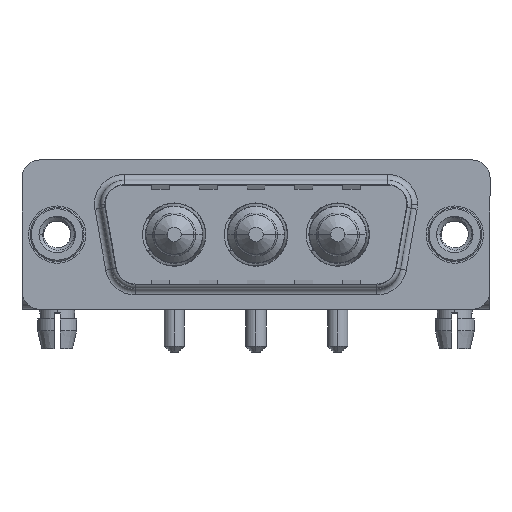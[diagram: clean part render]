
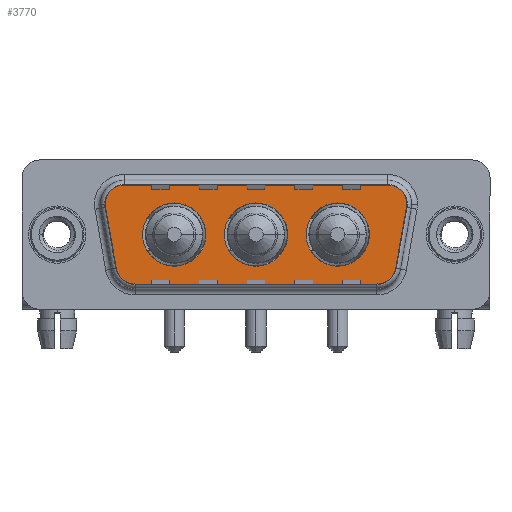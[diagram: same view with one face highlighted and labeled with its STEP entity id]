
A CAD part, top view. The second image highlights one B-rep face of the part: STEP entity #3770.
In plain terms, the highlighted planar face has unit normal (0, 0, 1).
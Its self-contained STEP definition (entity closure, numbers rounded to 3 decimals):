
#85 = ORIENTED_EDGE ( 'NONE', *, *, #2186, .F. ) ;
#625 = CARTESIAN_POINT ( 'NONE',  ( 9.8, 0., 0. ) ) ;
#735 = VERTEX_POINT ( 'NONE', #15365 ) ;
#1030 = EDGE_CURVE ( 'NONE', #1606, #735, #15286, .T. ) ;
#1065 = DIRECTION ( 'NONE',  ( 1., 0., 0. ) ) ;
#1342 = FACE_BOUND ( 'NONE', #11283, .T. ) ;
#1445 = AXIS2_PLACEMENT_3D ( 'NONE', #7161, #4649, #10979 ) ;
#1456 = CIRCLE ( 'NONE', #2249, 2.65 ) ;
#1606 = VERTEX_POINT ( 'NONE', #9211 ) ;
#1684 = CIRCLE ( 'NONE', #14431, 2. ) ;
#1829 = AXIS2_PLACEMENT_3D ( 'NONE', #4840, #5938, #9615 ) ;
#1981 = DIRECTION ( 'NONE',  ( 0., 0., 1. ) ) ;
#2066 = VERTEX_POINT ( 'NONE', #7993 ) ;
#2160 = CARTESIAN_POINT ( 'NONE',  ( 27.889, 2.9, 0. ) ) ;
#2186 = EDGE_CURVE ( 'NONE', #2377, #3686, #1456, .T. ) ;
#2249 = AXIS2_PLACEMENT_3D ( 'NONE', #7231, #9647, #12384 ) ;
#2377 = VERTEX_POINT ( 'NONE', #6630 ) ;
#2393 = CARTESIAN_POINT ( 'NONE',  ( 5.411, 4.9, 0. ) ) ;
#2565 = CARTESIAN_POINT ( 'NONE',  ( 3.441, 2.553, 0. ) ) ;
#2574 = EDGE_CURVE ( 'NONE', #12888, #13964, #14558, .T. ) ;
#2605 = AXIS2_PLACEMENT_3D ( 'NONE', #11259, #8933, #4928 ) ;
#2860 = VERTEX_POINT ( 'NONE', #3938 ) ;
#3021 = VECTOR ( 'NONE', #8652, 1000. ) ;
#3171 = CIRCLE ( 'NONE', #12470, 2.65 ) ;
#3242 = CARTESIAN_POINT ( 'NONE',  ( 12.45, 0., 0. ) ) ;
#3439 = CARTESIAN_POINT ( 'NONE',  ( 16.65, 0., 0. ) ) ;
#3446 = VERTEX_POINT ( 'NONE', #8181 ) ;
#3481 = LINE ( 'NONE', #2393, #12725 ) ;
#3588 = EDGE_CURVE ( 'NONE', #13690, #2066, #3481, .T. ) ;
#3669 = EDGE_CURVE ( 'NONE', #12091, #10074, #16150, .T. ) ;
#3686 = VERTEX_POINT ( 'NONE', #5006 ) ;
#3770 = ADVANCED_FACE ( 'NONE', ( #1342, #7768, #10258, #6184 ), #8850, .T. ) ;
#3938 = CARTESIAN_POINT ( 'NONE',  ( 28.836, -3.247, 0. ) ) ;
#4095 = CIRCLE ( 'NONE', #13646, 2.65 ) ;
#4265 = ORIENTED_EDGE ( 'NONE', *, *, #12433, .T. ) ;
#4649 = DIRECTION ( 'NONE',  ( 0., 0., 1. ) ) ;
#4803 = LINE ( 'NONE', #12307, #3021 ) ;
#4836 = ORIENTED_EDGE ( 'NONE', *, *, #1030, .F. ) ;
#4840 = CARTESIAN_POINT ( 'NONE',  ( 6.434, -2.9, 0. ) ) ;
#4928 = DIRECTION ( 'NONE',  ( 1., 0., 0. ) ) ;
#5006 = CARTESIAN_POINT ( 'NONE',  ( 20.85, 0., 0. ) ) ;
#5011 = CIRCLE ( 'NONE', #14308, 2. ) ;
#5017 = EDGE_CURVE ( 'NONE', #735, #1606, #3171, .T. ) ;
#5378 = ORIENTED_EDGE ( 'NONE', *, *, #3588, .T. ) ;
#5658 = DIRECTION ( 'NONE',  ( 1., 0., 0. ) ) ;
#5778 = DIRECTION ( 'NONE',  ( 1., 0., 0. ) ) ;
#5938 = DIRECTION ( 'NONE',  ( 0., 0., 1. ) ) ;
#5950 = EDGE_CURVE ( 'NONE', #10667, #3446, #7310, .T. ) ;
#6184 = FACE_OUTER_BOUND ( 'NONE', #13105, .T. ) ;
#6630 = CARTESIAN_POINT ( 'NONE',  ( 26.15, 0., 0. ) ) ;
#6725 = ORIENTED_EDGE ( 'NONE', *, *, #10808, .F. ) ;
#6967 = CARTESIAN_POINT ( 'NONE',  ( 27.889, 2.9, 0. ) ) ;
#7145 = AXIS2_PLACEMENT_3D ( 'NONE', #625, #15829, #13033 ) ;
#7161 = CARTESIAN_POINT ( 'NONE',  ( 23.5, 0., 0. ) ) ;
#7231 = CARTESIAN_POINT ( 'NONE',  ( 23.5, 0., 0. ) ) ;
#7310 = CIRCLE ( 'NONE', #12353, 2. ) ;
#7404 = DIRECTION ( 'NONE',  ( 0.174, -0.985, 0. ) ) ;
#7440 = CARTESIAN_POINT ( 'NONE',  ( 9.8, 0., 0. ) ) ;
#7768 = FACE_BOUND ( 'NONE', #12146, .T. ) ;
#7993 = CARTESIAN_POINT ( 'NONE',  ( 5.411, 4.9, 0. ) ) ;
#8053 = DIRECTION ( 'NONE',  ( 0., 0., 1. ) ) ;
#8173 = VERTEX_POINT ( 'NONE', #14516 ) ;
#8181 = CARTESIAN_POINT ( 'NONE',  ( 29.889, 2.9, 0. ) ) ;
#8199 = ORIENTED_EDGE ( 'NONE', *, *, #9866, .T. ) ;
#8332 = ORIENTED_EDGE ( 'NONE', *, *, #10462, .T. ) ;
#8424 = DIRECTION ( 'NONE',  ( 0., 0., 1. ) ) ;
#8535 = DIRECTION ( 'NONE',  ( 0., 0., 1. ) ) ;
#8571 = DIRECTION ( 'NONE',  ( -1., 0., 0. ) ) ;
#8586 = DIRECTION ( 'NONE',  ( -1., 0., 0. ) ) ;
#8592 = CARTESIAN_POINT ( 'NONE',  ( 5.411, 2.9, 0. ) ) ;
#8652 = DIRECTION ( 'NONE',  ( 1., 0., 0. ) ) ;
#8850 = PLANE ( 'NONE',  #2605 ) ;
#8933 = DIRECTION ( 'NONE',  ( 0., 0., 1. ) ) ;
#9126 = LINE ( 'NONE', #15313, #11811 ) ;
#9205 = EDGE_CURVE ( 'NONE', #2066, #11883, #16244, .T. ) ;
#9211 = CARTESIAN_POINT ( 'NONE',  ( 19.3, 0., 0. ) ) ;
#9243 = CARTESIAN_POINT ( 'NONE',  ( 4.464, -3.247, 0. ) ) ;
#9438 = ORIENTED_EDGE ( 'NONE', *, *, #5950, .T. ) ;
#9507 = EDGE_CURVE ( 'NONE', #3446, #13690, #1684, .T. ) ;
#9532 = CARTESIAN_POINT ( 'NONE',  ( 29.859, 2.553, 0. ) ) ;
#9570 = CARTESIAN_POINT ( 'NONE',  ( 26.866, -2.9, 0. ) ) ;
#9615 = DIRECTION ( 'NONE',  ( -1., 0., 0. ) ) ;
#9647 = DIRECTION ( 'NONE',  ( 0., 0., 1. ) ) ;
#9866 = EDGE_CURVE ( 'NONE', #10074, #8173, #4803, .T. ) ;
#10074 = VERTEX_POINT ( 'NONE', #15837 ) ;
#10258 = FACE_BOUND ( 'NONE', #10494, .T. ) ;
#10366 = DIRECTION ( 'NONE',  ( 0.174, 0.985, 0. ) ) ;
#10397 = ORIENTED_EDGE ( 'NONE', *, *, #9507, .T. ) ;
#10462 = EDGE_CURVE ( 'NONE', #2860, #10667, #9126, .T. ) ;
#10494 = EDGE_LOOP ( 'NONE', ( #6725, #14562 ) ) ;
#10601 = ORIENTED_EDGE ( 'NONE', *, *, #11227, .F. ) ;
#10667 = VERTEX_POINT ( 'NONE', #9532 ) ;
#10684 = ORIENTED_EDGE ( 'NONE', *, *, #11315, .T. ) ;
#10787 = DIRECTION ( 'NONE',  ( -1., 0., 0. ) ) ;
#10808 = EDGE_CURVE ( 'NONE', #13964, #12888, #4095, .T. ) ;
#10979 = DIRECTION ( 'NONE',  ( 1., 0., 0. ) ) ;
#11064 = CARTESIAN_POINT ( 'NONE',  ( 16.65, 0., 0. ) ) ;
#11159 = CARTESIAN_POINT ( 'NONE',  ( 27.889, 4.9, 0. ) ) ;
#11227 = EDGE_CURVE ( 'NONE', #3686, #2377, #15767, .T. ) ;
#11259 = CARTESIAN_POINT ( 'NONE',  ( 26.866, -2.9, 0. ) ) ;
#11283 = EDGE_LOOP ( 'NONE', ( #4836, #11346 ) ) ;
#11315 = EDGE_CURVE ( 'NONE', #11883, #12091, #13871, .T. ) ;
#11346 = ORIENTED_EDGE ( 'NONE', *, *, #5017, .F. ) ;
#11513 = CARTESIAN_POINT ( 'NONE',  ( 3.441, 2.553, 0. ) ) ;
#11811 = VECTOR ( 'NONE', #10366, 1000. ) ;
#11883 = VERTEX_POINT ( 'NONE', #11513 ) ;
#12091 = VERTEX_POINT ( 'NONE', #9243 ) ;
#12146 = EDGE_LOOP ( 'NONE', ( #85, #10601 ) ) ;
#12307 = CARTESIAN_POINT ( 'NONE',  ( 6.434, -4.9, 0. ) ) ;
#12353 = AXIS2_PLACEMENT_3D ( 'NONE', #2160, #13472, #8586 ) ;
#12384 = DIRECTION ( 'NONE',  ( 1., 0., 0. ) ) ;
#12433 = EDGE_CURVE ( 'NONE', #8173, #2860, #5011, .T. ) ;
#12470 = AXIS2_PLACEMENT_3D ( 'NONE', #3439, #8535, #13585 ) ;
#12510 = DIRECTION ( 'NONE',  ( 0., 0., 1. ) ) ;
#12725 = VECTOR ( 'NONE', #8571, 1000. ) ;
#12888 = VERTEX_POINT ( 'NONE', #14092 ) ;
#12932 = AXIS2_PLACEMENT_3D ( 'NONE', #11064, #13624, #1065 ) ;
#13033 = DIRECTION ( 'NONE',  ( 1., 0., 0. ) ) ;
#13049 = ORIENTED_EDGE ( 'NONE', *, *, #9205, .T. ) ;
#13097 = AXIS2_PLACEMENT_3D ( 'NONE', #8592, #8424, #16033 ) ;
#13105 = EDGE_LOOP ( 'NONE', ( #4265, #8332, #9438, #10397, #5378, #13049, #10684, #16422, #8199 ) ) ;
#13472 = DIRECTION ( 'NONE',  ( 0., 0., 1. ) ) ;
#13585 = DIRECTION ( 'NONE',  ( 1., 0., 0. ) ) ;
#13624 = DIRECTION ( 'NONE',  ( 0., 0., 1. ) ) ;
#13646 = AXIS2_PLACEMENT_3D ( 'NONE', #7440, #12510, #5778 ) ;
#13690 = VERTEX_POINT ( 'NONE', #11159 ) ;
#13871 = LINE ( 'NONE', #2565, #15729 ) ;
#13964 = VERTEX_POINT ( 'NONE', #3242 ) ;
#14092 = CARTESIAN_POINT ( 'NONE',  ( 7.15, 0., 0. ) ) ;
#14308 = AXIS2_PLACEMENT_3D ( 'NONE', #9570, #1981, #5658 ) ;
#14431 = AXIS2_PLACEMENT_3D ( 'NONE', #6967, #8053, #10787 ) ;
#14516 = CARTESIAN_POINT ( 'NONE',  ( 26.866, -4.9, 0. ) ) ;
#14558 = CIRCLE ( 'NONE', #7145, 2.65 ) ;
#14562 = ORIENTED_EDGE ( 'NONE', *, *, #2574, .F. ) ;
#15286 = CIRCLE ( 'NONE', #12932, 2.65 ) ;
#15313 = CARTESIAN_POINT ( 'NONE',  ( 29.859, 2.553, 0. ) ) ;
#15365 = CARTESIAN_POINT ( 'NONE',  ( 14., 0., 0. ) ) ;
#15729 = VECTOR ( 'NONE', #7404, 1000. ) ;
#15767 = CIRCLE ( 'NONE', #1445, 2.65 ) ;
#15829 = DIRECTION ( 'NONE',  ( 0., 0., 1. ) ) ;
#15837 = CARTESIAN_POINT ( 'NONE',  ( 6.434, -4.9, 0. ) ) ;
#16033 = DIRECTION ( 'NONE',  ( 1., 0., 0. ) ) ;
#16150 = CIRCLE ( 'NONE', #1829, 2. ) ;
#16244 = CIRCLE ( 'NONE', #13097, 2. ) ;
#16422 = ORIENTED_EDGE ( 'NONE', *, *, #3669, .T. ) ;
